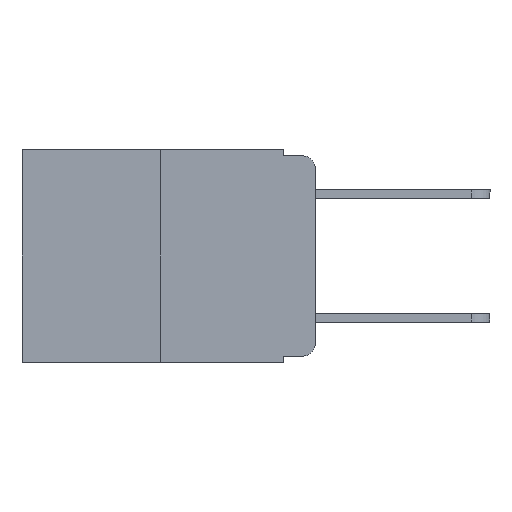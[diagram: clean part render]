
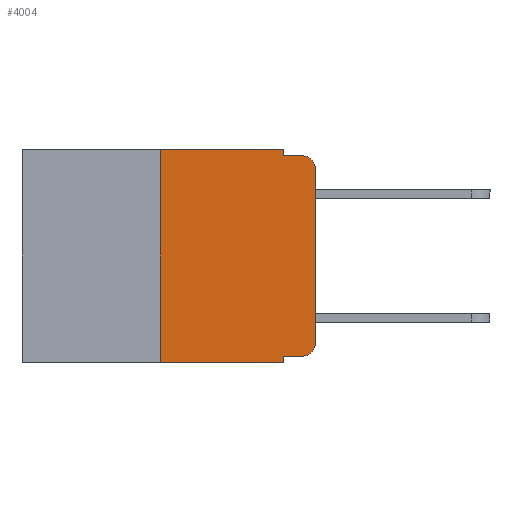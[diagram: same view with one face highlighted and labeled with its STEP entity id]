
A CAD part, left-side view. The second image highlights one B-rep face of the part: STEP entity #4004.
In plain terms, the highlighted planar face has unit normal (-1, 0, 0).
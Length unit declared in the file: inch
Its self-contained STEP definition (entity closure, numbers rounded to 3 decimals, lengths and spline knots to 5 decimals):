
#27 = ORIENTED_EDGE ( 'NONE', *, *, #9056, .F. ) ;
#176 = AXIS2_PLACEMENT_3D ( 'NONE', #346, #3275, #10000 ) ;
#287 = CIRCLE ( 'NONE', #2936, 0.02 ) ;
#336 = CARTESIAN_POINT ( 'NONE',  ( 0., 0.051, -0.01 ) ) ;
#346 = CARTESIAN_POINT ( 'NONE',  ( 0., 0.02, -0.03 ) ) ;
#612 = PLANE ( 'NONE',  #5939 ) ;
#624 = DIRECTION ( 'NONE',  ( -1., 0., 0. ) ) ;
#660 = EDGE_CURVE ( 'NONE', #9815, #4722, #10462, .T. ) ;
#699 = VERTEX_POINT ( 'NONE', #9766 ) ;
#1045 = EDGE_LOOP ( 'NONE', ( #6498, #5990, #3816, #2162, #27, #7151, #2990, #9999, #4598, #7625 ) ) ;
#1304 = EDGE_CURVE ( 'NONE', #6968, #5531, #1654, .T. ) ;
#1471 = DIRECTION ( 'NONE',  ( 0., -1., 0. ) ) ;
#1654 = LINE ( 'NONE', #9660, #7933 ) ;
#1716 = CARTESIAN_POINT ( 'NONE',  ( 0., 0.02, -0.313 ) ) ;
#2162 = ORIENTED_EDGE ( 'NONE', *, *, #2871, .F. ) ;
#2373 = EDGE_CURVE ( 'NONE', #5531, #699, #287, .T. ) ;
#2842 = CARTESIAN_POINT ( 'NONE',  ( 0., 0.051, 0. ) ) ;
#2871 = EDGE_CURVE ( 'NONE', #6303, #6872, #3849, .T. ) ;
#2874 = CARTESIAN_POINT ( 'NONE',  ( 0., 0.051, 0. ) ) ;
#2936 = AXIS2_PLACEMENT_3D ( 'NONE', #1716, #624, #4490 ) ;
#2990 = ORIENTED_EDGE ( 'NONE', *, *, #3179, .T. ) ;
#3179 = EDGE_CURVE ( 'NONE', #5799, #4917, #11451, .T. ) ;
#3275 = DIRECTION ( 'NONE',  ( -1., 0., 0. ) ) ;
#3315 = VECTOR ( 'NONE', #1471, 39.37008 ) ;
#3790 = CARTESIAN_POINT ( 'NONE',  ( 0., 0., -0.03 ) ) ;
#3816 = ORIENTED_EDGE ( 'NONE', *, *, #10228, .F. ) ;
#3849 = LINE ( 'NONE', #2842, #11097 ) ;
#3855 = CARTESIAN_POINT ( 'NONE',  ( 0., 0.02, -0.333 ) ) ;
#4004 = ADVANCED_FACE ( 'NONE', ( #4476 ), #612, .F. ) ;
#4302 = VECTOR ( 'NONE', #8924, 39.37008 ) ;
#4451 = DIRECTION ( 'NONE',  ( 0., 0., -1. ) ) ;
#4461 = LINE ( 'NONE', #9179, #11493 ) ;
#4476 = FACE_OUTER_BOUND ( 'NONE', #1045, .T. ) ;
#4490 = DIRECTION ( 'NONE',  ( 0., 0., -1. ) ) ;
#4504 = EDGE_CURVE ( 'NONE', #5799, #10864, #4461, .T. ) ;
#4598 = ORIENTED_EDGE ( 'NONE', *, *, #1304, .T. ) ;
#4675 = DIRECTION ( 'NONE',  ( 0., 0., -1. ) ) ;
#4722 = VERTEX_POINT ( 'NONE', #12403 ) ;
#4870 = CARTESIAN_POINT ( 'NONE',  ( 0., 0., 0. ) ) ;
#4883 = EDGE_CURVE ( 'NONE', #6968, #4917, #10309, .T. ) ;
#4885 = VECTOR ( 'NONE', #7227, 39.37008 ) ;
#4917 = VERTEX_POINT ( 'NONE', #12269 ) ;
#5510 = DIRECTION ( 'NONE',  ( 0., -1., 0. ) ) ;
#5531 = VERTEX_POINT ( 'NONE', #3855 ) ;
#5799 = VERTEX_POINT ( 'NONE', #9182 ) ;
#5929 = CARTESIAN_POINT ( 'NONE',  ( 0., 0.051, -0.333 ) ) ;
#5939 = AXIS2_PLACEMENT_3D ( 'NONE', #9455, #7492, #4675 ) ;
#5990 = ORIENTED_EDGE ( 'NONE', *, *, #660, .T. ) ;
#6303 = VERTEX_POINT ( 'NONE', #2874 ) ;
#6498 = ORIENTED_EDGE ( 'NONE', *, *, #7207, .T. ) ;
#6872 = VERTEX_POINT ( 'NONE', #7630 ) ;
#6968 = VERTEX_POINT ( 'NONE', #5929 ) ;
#7091 = CARTESIAN_POINT ( 'NONE',  ( 0., 0.473, 0. ) ) ;
#7151 = ORIENTED_EDGE ( 'NONE', *, *, #4504, .F. ) ;
#7207 = EDGE_CURVE ( 'NONE', #699, #9815, #8562, .T. ) ;
#7227 = DIRECTION ( 'NONE',  ( 0., -1., 0. ) ) ;
#7289 = DIRECTION ( 'NONE',  ( 0., 0., 1. ) ) ;
#7492 = DIRECTION ( 'NONE',  ( 1., 0., 0. ) ) ;
#7625 = ORIENTED_EDGE ( 'NONE', *, *, #2373, .T. ) ;
#7630 = CARTESIAN_POINT ( 'NONE',  ( 0., 0.051, -0.01 ) ) ;
#7933 = VECTOR ( 'NONE', #5510, 39.37008 ) ;
#8340 = CARTESIAN_POINT ( 'NONE',  ( 0., 0.051, 0. ) ) ;
#8538 = CARTESIAN_POINT ( 'NONE',  ( 0., 0.473, -0.343 ) ) ;
#8562 = LINE ( 'NONE', #4870, #10314 ) ;
#8924 = DIRECTION ( 'NONE',  ( 0., -1., 0. ) ) ;
#9056 = EDGE_CURVE ( 'NONE', #10864, #6303, #9866, .T. ) ;
#9179 = CARTESIAN_POINT ( 'NONE',  ( 0., 0.25, 0. ) ) ;
#9182 = CARTESIAN_POINT ( 'NONE',  ( 0., 0.25, -0.343 ) ) ;
#9455 = CARTESIAN_POINT ( 'NONE',  ( 0., 0.473, 0. ) ) ;
#9660 = CARTESIAN_POINT ( 'NONE',  ( 0., 0.051, -0.333 ) ) ;
#9713 = DIRECTION ( 'NONE',  ( 0., 0., 1. ) ) ;
#9766 = CARTESIAN_POINT ( 'NONE',  ( 0., 0., -0.313 ) ) ;
#9804 = VECTOR ( 'NONE', #4451, 39.37008 ) ;
#9815 = VERTEX_POINT ( 'NONE', #3790 ) ;
#9866 = LINE ( 'NONE', #7091, #4302 ) ;
#9929 = LINE ( 'NONE', #336, #3315 ) ;
#9999 = ORIENTED_EDGE ( 'NONE', *, *, #4883, .F. ) ;
#10000 = DIRECTION ( 'NONE',  ( 0., 0., -1. ) ) ;
#10228 = EDGE_CURVE ( 'NONE', #6872, #4722, #9929, .T. ) ;
#10309 = LINE ( 'NONE', #8340, #9804 ) ;
#10314 = VECTOR ( 'NONE', #9713, 39.37008 ) ;
#10462 = CIRCLE ( 'NONE', #176, 0.02 ) ;
#10864 = VERTEX_POINT ( 'NONE', #11751 ) ;
#11097 = VECTOR ( 'NONE', #11417, 39.37008 ) ;
#11417 = DIRECTION ( 'NONE',  ( 0., 0., -1. ) ) ;
#11451 = LINE ( 'NONE', #8538, #4885 ) ;
#11493 = VECTOR ( 'NONE', #7289, 39.37008 ) ;
#11751 = CARTESIAN_POINT ( 'NONE',  ( 0., 0.25, 0. ) ) ;
#12269 = CARTESIAN_POINT ( 'NONE',  ( 0., 0.051, -0.343 ) ) ;
#12403 = CARTESIAN_POINT ( 'NONE',  ( 0., 0.02, -0.01 ) ) ;
